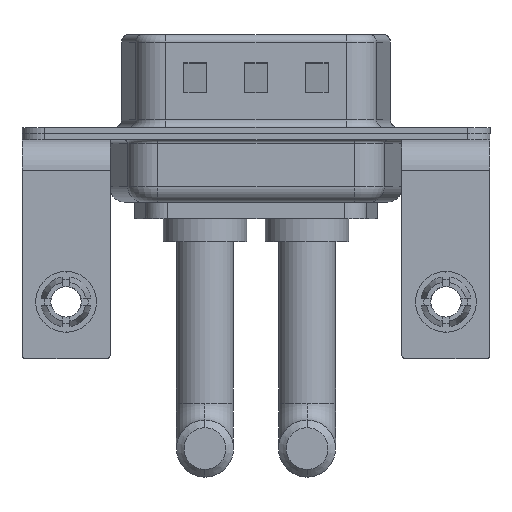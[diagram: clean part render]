
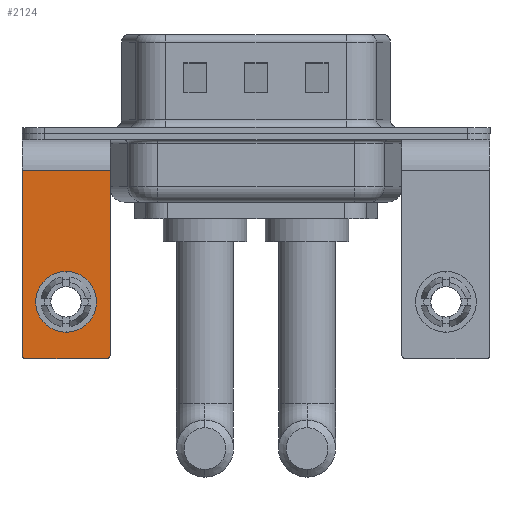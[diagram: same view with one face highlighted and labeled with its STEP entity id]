
A CAD part, front view. The second image highlights one B-rep face of the part: STEP entity #2124.
In plain terms, the highlighted planar face has unit normal (0, -1, 0).
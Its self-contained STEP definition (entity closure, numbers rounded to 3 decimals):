
#242 = ORIENTED_EDGE ( 'NONE', *, *, #7229, .T. ) ;
#337 = PLANE ( 'NONE',  #16209 ) ;
#413 = DIRECTION ( 'NONE',  ( 0., 0., -1. ) ) ;
#1180 = CARTESIAN_POINT ( 'NONE',  ( 2.9, -6.25, -2.4 ) ) ;
#1265 = EDGE_LOOP ( 'NONE', ( #2825, #3051, #3897, #7616, #4896, #242 ) ) ;
#1361 = CARTESIAN_POINT ( 'NONE',  ( 2.9, -6.25, -2.4 ) ) ;
#1509 = EDGE_CURVE ( 'NONE', #10094, #16088, #2238, .T. ) ;
#1637 = LINE ( 'NONE', #16888, #15796 ) ;
#1841 = CARTESIAN_POINT ( 'NONE',  ( 2.65, -6.25, -14.8 ) ) ;
#2124 = ADVANCED_FACE ( 'NONE', ( #9499, #11894 ), #337, .F. ) ;
#2238 = CIRCLE ( 'NONE', #13994, 2. ) ;
#2277 = DIRECTION ( 'NONE',  ( 0., -1., 0. ) ) ;
#2299 = CIRCLE ( 'NONE', #10773, 0.25 ) ;
#2729 = DIRECTION ( 'NONE',  ( 0., 0., 1. ) ) ;
#2805 = VECTOR ( 'NONE', #12097, 1000. ) ;
#2825 = ORIENTED_EDGE ( 'NONE', *, *, #14095, .T. ) ;
#2831 = LINE ( 'NONE', #10634, #2805 ) ;
#2906 = EDGE_CURVE ( 'NONE', #11012, #6164, #2831, .T. ) ;
#3051 = ORIENTED_EDGE ( 'NONE', *, *, #9379, .T. ) ;
#3897 = ORIENTED_EDGE ( 'NONE', *, *, #2906, .F. ) ;
#4127 = CARTESIAN_POINT ( 'NONE',  ( 2.9, -6.25, -2.4 ) ) ;
#4815 = EDGE_CURVE ( 'NONE', #11012, #6443, #2299, .T. ) ;
#4896 = ORIENTED_EDGE ( 'NONE', *, *, #16149, .F. ) ;
#5245 = DIRECTION ( 'NONE',  ( 0., 0., -1. ) ) ;
#5441 = VECTOR ( 'NONE', #413, 1000. ) ;
#5700 = VECTOR ( 'NONE', #6426, 1000. ) ;
#5908 = CARTESIAN_POINT ( 'NONE',  ( 2.9, -6.25, -2.4 ) ) ;
#6164 = VERTEX_POINT ( 'NONE', #6595 ) ;
#6299 = CARTESIAN_POINT ( 'NONE',  ( 0., -6.25, -11.07 ) ) ;
#6406 = CARTESIAN_POINT ( 'NONE',  ( -2.65, -6.25, -14.55 ) ) ;
#6426 = DIRECTION ( 'NONE',  ( -1., 0., 0. ) ) ;
#6443 = VERTEX_POINT ( 'NONE', #11932 ) ;
#6461 = DIRECTION ( 'NONE',  ( 0., 0., 1. ) ) ;
#6595 = CARTESIAN_POINT ( 'NONE',  ( -2.65, -6.25, -14.8 ) ) ;
#6729 = DIRECTION ( 'NONE',  ( 0., 1., 0. ) ) ;
#7228 = ORIENTED_EDGE ( 'NONE', *, *, #15792, .T. ) ;
#7229 = EDGE_CURVE ( 'NONE', #14159, #12935, #10097, .T. ) ;
#7616 = ORIENTED_EDGE ( 'NONE', *, *, #4815, .T. ) ;
#8626 = DIRECTION ( 'NONE',  ( 0., -1., 0. ) ) ;
#9379 = EDGE_CURVE ( 'NONE', #15800, #6164, #10928, .T. ) ;
#9499 = FACE_BOUND ( 'NONE', #9558, .T. ) ;
#9558 = EDGE_LOOP ( 'NONE', ( #7228, #13497 ) ) ;
#10094 = VERTEX_POINT ( 'NONE', #13600 ) ;
#10097 = LINE ( 'NONE', #1180, #5700 ) ;
#10611 = AXIS2_PLACEMENT_3D ( 'NONE', #13306, #6729, #14588 ) ;
#10634 = CARTESIAN_POINT ( 'NONE',  ( 2.9, -6.25, -14.8 ) ) ;
#10773 = AXIS2_PLACEMENT_3D ( 'NONE', #16418, #8626, #13829 ) ;
#10928 = CIRCLE ( 'NONE', #15312, 0.25 ) ;
#11012 = VERTEX_POINT ( 'NONE', #1841 ) ;
#11614 = DIRECTION ( 'NONE',  ( 0., 0., 1. ) ) ;
#11894 = FACE_OUTER_BOUND ( 'NONE', #1265, .T. ) ;
#11932 = CARTESIAN_POINT ( 'NONE',  ( 2.9, -6.25, -14.55 ) ) ;
#12034 = CARTESIAN_POINT ( 'NONE',  ( -2.9, -6.25, -14.55 ) ) ;
#12097 = DIRECTION ( 'NONE',  ( -1., 0., 0. ) ) ;
#12232 = LINE ( 'NONE', #5908, #5441 ) ;
#12868 = DIRECTION ( 'NONE',  ( 0., 1., 0. ) ) ;
#12935 = VERTEX_POINT ( 'NONE', #13845 ) ;
#13306 = CARTESIAN_POINT ( 'NONE',  ( 0., -6.25, -11.07 ) ) ;
#13497 = ORIENTED_EDGE ( 'NONE', *, *, #1509, .T. ) ;
#13600 = CARTESIAN_POINT ( 'NONE',  ( 0., -6.25, -9.07 ) ) ;
#13829 = DIRECTION ( 'NONE',  ( 0., 0., 1. ) ) ;
#13845 = CARTESIAN_POINT ( 'NONE',  ( -2.9, -6.25, -2.4 ) ) ;
#13884 = CIRCLE ( 'NONE', #10611, 2. ) ;
#13994 = AXIS2_PLACEMENT_3D ( 'NONE', #6299, #12868, #6461 ) ;
#14095 = EDGE_CURVE ( 'NONE', #12935, #15800, #1637, .T. ) ;
#14159 = VERTEX_POINT ( 'NONE', #4127 ) ;
#14588 = DIRECTION ( 'NONE',  ( 0., 0., 1. ) ) ;
#15312 = AXIS2_PLACEMENT_3D ( 'NONE', #6406, #2277, #11614 ) ;
#15432 = CARTESIAN_POINT ( 'NONE',  ( 0., -6.25, -13.07 ) ) ;
#15792 = EDGE_CURVE ( 'NONE', #16088, #10094, #13884, .T. ) ;
#15796 = VECTOR ( 'NONE', #5245, 1000. ) ;
#15800 = VERTEX_POINT ( 'NONE', #12034 ) ;
#16002 = DIRECTION ( 'NONE',  ( 0., 1., 0. ) ) ;
#16088 = VERTEX_POINT ( 'NONE', #15432 ) ;
#16149 = EDGE_CURVE ( 'NONE', #14159, #6443, #12232, .T. ) ;
#16209 = AXIS2_PLACEMENT_3D ( 'NONE', #1361, #16002, #2729 ) ;
#16418 = CARTESIAN_POINT ( 'NONE',  ( 2.65, -6.25, -14.55 ) ) ;
#16888 = CARTESIAN_POINT ( 'NONE',  ( -2.9, -6.25, -2.4 ) ) ;
